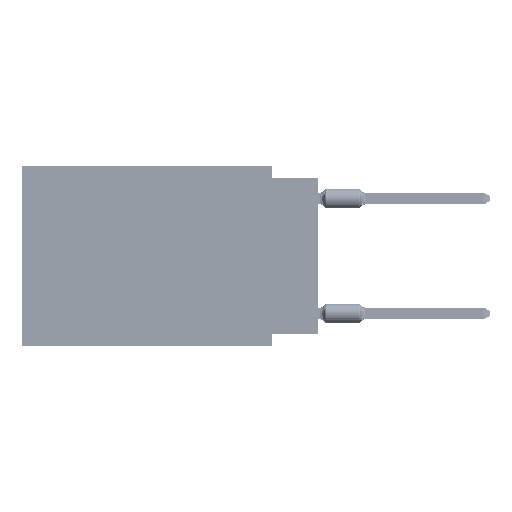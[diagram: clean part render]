
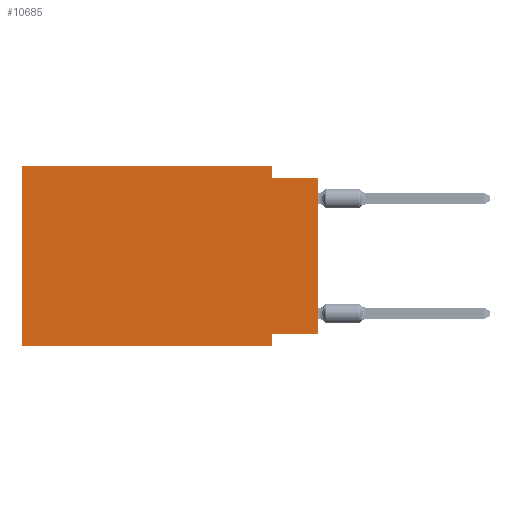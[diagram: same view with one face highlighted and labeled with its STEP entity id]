
A CAD part, left-side view. The second image highlights one B-rep face of the part: STEP entity #10685.
In plain terms, the highlighted planar face has unit normal (-1, 0, 0).
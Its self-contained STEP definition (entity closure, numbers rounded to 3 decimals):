
#1965 = LINE ( 'NONE', #36258, #29379 ) ;
#3726 = EDGE_LOOP ( 'NONE', ( #61193, #24931, #44804, #9559, #81705, #5719, #52922, #67527 ) ) ;
#4066 = CARTESIAN_POINT ( 'NONE',  ( 0., 16.383, 0. ) ) ;
#4187 = PLANE ( 'NONE',  #54474 ) ;
#4468 = LINE ( 'NONE', #12274, #50874 ) ;
#4721 = EDGE_CURVE ( 'NONE', #69539, #40599, #57480, .T. ) ;
#5719 = ORIENTED_EDGE ( 'NONE', *, *, #28599, .T. ) ;
#9445 = DIRECTION ( 'NONE',  ( 1., 0., 0. ) ) ;
#9468 = CARTESIAN_POINT ( 'NONE',  ( 0., 2.54, -9.906 ) ) ;
#9559 = ORIENTED_EDGE ( 'NONE', *, *, #4721, .F. ) ;
#10589 = DIRECTION ( 'NONE',  ( 0., -1., 0. ) ) ;
#10685 = ADVANCED_FACE ( 'NONE', ( #29417 ), #4187, .F. ) ;
#12274 = CARTESIAN_POINT ( 'NONE',  ( 0., 2.54, 0. ) ) ;
#14887 = CARTESIAN_POINT ( 'NONE',  ( 0., 0., -9.271 ) ) ;
#15705 = CARTESIAN_POINT ( 'NONE',  ( 0., 16.383, -9.906 ) ) ;
#15770 = LINE ( 'NONE', #67927, #82003 ) ;
#16163 = CARTESIAN_POINT ( 'NONE',  ( 0., 0., 0. ) ) ;
#16185 = CARTESIAN_POINT ( 'NONE',  ( 0., 2.54, -0.635 ) ) ;
#18765 = CARTESIAN_POINT ( 'NONE',  ( 0., 2.54, 0. ) ) ;
#20201 = CARTESIAN_POINT ( 'NONE',  ( 0., 16.383, 0. ) ) ;
#23495 = EDGE_CURVE ( 'NONE', #37125, #81443, #1965, .T. ) ;
#24931 = ORIENTED_EDGE ( 'NONE', *, *, #23495, .F. ) ;
#27534 = DIRECTION ( 'NONE',  ( 0., 0., -1. ) ) ;
#28599 = EDGE_CURVE ( 'NONE', #29445, #57649, #75232, .T. ) ;
#28627 = VERTEX_POINT ( 'NONE', #62191 ) ;
#29379 = VECTOR ( 'NONE', #68003, 1000. ) ;
#29417 = FACE_OUTER_BOUND ( 'NONE', #3726, .T. ) ;
#29445 = VERTEX_POINT ( 'NONE', #51050 ) ;
#29827 = DIRECTION ( 'NONE',  ( 0., 0., 1. ) ) ;
#34879 = DIRECTION ( 'NONE',  ( 0., 1., 0. ) ) ;
#35435 = CARTESIAN_POINT ( 'NONE',  ( 0., 0., -9.271 ) ) ;
#36258 = CARTESIAN_POINT ( 'NONE',  ( 0., 0., -0.635 ) ) ;
#36821 = VERTEX_POINT ( 'NONE', #35435 ) ;
#37125 = VERTEX_POINT ( 'NONE', #16185 ) ;
#38358 = DIRECTION ( 'NONE',  ( 0., 0., -1. ) ) ;
#40599 = VERTEX_POINT ( 'NONE', #18765 ) ;
#44804 = ORIENTED_EDGE ( 'NONE', *, *, #52624, .F. ) ;
#46276 = VECTOR ( 'NONE', #34879, 1000. ) ;
#48803 = EDGE_CURVE ( 'NONE', #36821, #28627, #74424, .T. ) ;
#48955 = CARTESIAN_POINT ( 'NONE',  ( 0., 16.383, 0. ) ) ;
#50874 = VECTOR ( 'NONE', #38358, 1000. ) ;
#51050 = CARTESIAN_POINT ( 'NONE',  ( 0., 16.383, -9.906 ) ) ;
#51366 = VECTOR ( 'NONE', #10589, 1000. ) ;
#52624 = EDGE_CURVE ( 'NONE', #40599, #37125, #4468, .T. ) ;
#52922 = ORIENTED_EDGE ( 'NONE', *, *, #81096, .F. ) ;
#54474 = AXIS2_PLACEMENT_3D ( 'NONE', #48955, #9445, #55893 ) ;
#55893 = DIRECTION ( 'NONE',  ( 0., 0., -1. ) ) ;
#56961 = EDGE_CURVE ( 'NONE', #36821, #81443, #75691, .T. ) ;
#57108 = VECTOR ( 'NONE', #69186, 1000. ) ;
#57480 = LINE ( 'NONE', #4066, #51366 ) ;
#57649 = VERTEX_POINT ( 'NONE', #9468 ) ;
#59403 = CARTESIAN_POINT ( 'NONE',  ( 0., 16.383, 0. ) ) ;
#60061 = VECTOR ( 'NONE', #29827, 1000. ) ;
#61193 = ORIENTED_EDGE ( 'NONE', *, *, #56961, .T. ) ;
#62191 = CARTESIAN_POINT ( 'NONE',  ( 0., 2.54, -9.271 ) ) ;
#67527 = ORIENTED_EDGE ( 'NONE', *, *, #48803, .F. ) ;
#67594 = VECTOR ( 'NONE', #68720, 1000. ) ;
#67927 = CARTESIAN_POINT ( 'NONE',  ( 0., 2.54, -9.906 ) ) ;
#68003 = DIRECTION ( 'NONE',  ( 0., -1., 0. ) ) ;
#68720 = DIRECTION ( 'NONE',  ( 0., -1., 0. ) ) ;
#69186 = DIRECTION ( 'NONE',  ( 0., 0., 1. ) ) ;
#69539 = VERTEX_POINT ( 'NONE', #20201 ) ;
#72447 = LINE ( 'NONE', #59403, #60061 ) ;
#74424 = LINE ( 'NONE', #14887, #46276 ) ;
#75232 = LINE ( 'NONE', #15705, #67594 ) ;
#75691 = LINE ( 'NONE', #16163, #57108 ) ;
#77100 = EDGE_CURVE ( 'NONE', #29445, #69539, #72447, .T. ) ;
#78689 = CARTESIAN_POINT ( 'NONE',  ( 0., 0., -0.635 ) ) ;
#81096 = EDGE_CURVE ( 'NONE', #28627, #57649, #15770, .T. ) ;
#81443 = VERTEX_POINT ( 'NONE', #78689 ) ;
#81705 = ORIENTED_EDGE ( 'NONE', *, *, #77100, .F. ) ;
#82003 = VECTOR ( 'NONE', #27534, 1000. ) ;
